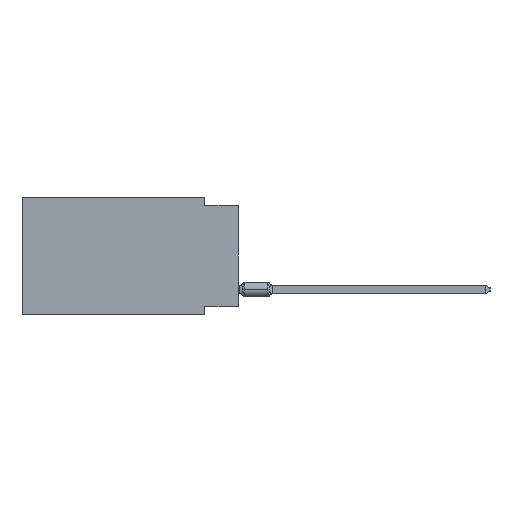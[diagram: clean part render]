
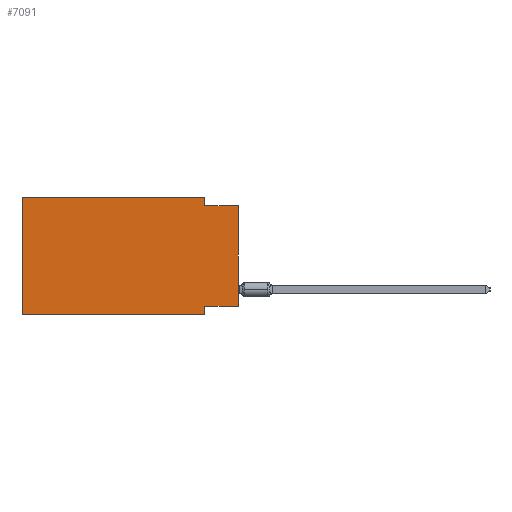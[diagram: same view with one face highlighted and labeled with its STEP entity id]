
A CAD part, left-side view. The second image highlights one B-rep face of the part: STEP entity #7091.
In plain terms, the highlighted planar face has unit normal (-1, 0, 0).
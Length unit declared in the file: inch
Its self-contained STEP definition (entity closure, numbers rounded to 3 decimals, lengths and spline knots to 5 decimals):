
#1363 = CARTESIAN_POINT ( 'NONE',  ( 0., 0., -0.325 ) ) ;
#2406 = DIRECTION ( 'NONE',  ( 0., 0., -1. ) ) ;
#4223 = EDGE_CURVE ( 'NONE', #99564, #10170, #31733, .T. ) ;
#4282 = LINE ( 'NONE', #84194, #91702 ) ;
#7091 = ADVANCED_FACE ( 'NONE', ( #85980 ), #93280, .F. ) ;
#7467 = CARTESIAN_POINT ( 'NONE',  ( 0., 0.645, 0. ) ) ;
#8281 = LINE ( 'NONE', #88220, #32033 ) ;
#8708 = EDGE_CURVE ( 'NONE', #79408, #15203, #8281, .T. ) ;
#10170 = VERTEX_POINT ( 'NONE', #73084 ) ;
#10191 = CARTESIAN_POINT ( 'NONE',  ( 0., 0.1, 0. ) ) ;
#11594 = CARTESIAN_POINT ( 'NONE',  ( 0., 0., 0. ) ) ;
#12178 = EDGE_CURVE ( 'NONE', #32904, #79408, #102466, .T. ) ;
#15203 = VERTEX_POINT ( 'NONE', #91053 ) ;
#17018 = VERTEX_POINT ( 'NONE', #29760 ) ;
#17642 = DIRECTION ( 'NONE',  ( 0., -1., 0. ) ) ;
#20343 = CARTESIAN_POINT ( 'NONE',  ( 0., 0.1, -0.025 ) ) ;
#28086 = VECTOR ( 'NONE', #47106, 39.37008 ) ;
#29302 = ORIENTED_EDGE ( 'NONE', *, *, #82862, .F. ) ;
#29760 = CARTESIAN_POINT ( 'NONE',  ( 0., 0.1, -0.325 ) ) ;
#31733 = LINE ( 'NONE', #101323, #88488 ) ;
#31818 = DIRECTION ( 'NONE',  ( 0., -1., 0. ) ) ;
#32033 = VECTOR ( 'NONE', #31818, 39.37008 ) ;
#32904 = VERTEX_POINT ( 'NONE', #97668 ) ;
#39822 = LINE ( 'NONE', #1363, #28086 ) ;
#40820 = ORIENTED_EDGE ( 'NONE', *, *, #8708, .F. ) ;
#44756 = DIRECTION ( 'NONE',  ( 0., 0., -1. ) ) ;
#45293 = ORIENTED_EDGE ( 'NONE', *, *, #4223, .F. ) ;
#47106 = DIRECTION ( 'NONE',  ( 0., 1., 0. ) ) ;
#51353 = EDGE_CURVE ( 'NONE', #32904, #85572, #88753, .T. ) ;
#53718 = EDGE_CURVE ( 'NONE', #17018, #85572, #4282, .T. ) ;
#54273 = ORIENTED_EDGE ( 'NONE', *, *, #85349, .T. ) ;
#63018 = DIRECTION ( 'NONE',  ( 0., 0., 1. ) ) ;
#63971 = ORIENTED_EDGE ( 'NONE', *, *, #53718, .F. ) ;
#66106 = DIRECTION ( 'NONE',  ( 0., 0., 1. ) ) ;
#66278 = LINE ( 'NONE', #10191, #70464 ) ;
#68367 = VECTOR ( 'NONE', #17642, 39.37008 ) ;
#68735 = CARTESIAN_POINT ( 'NONE',  ( 0., 0., -0.325 ) ) ;
#70464 = VECTOR ( 'NONE', #2406, 39.37008 ) ;
#70679 = DIRECTION ( 'NONE',  ( 0., -1., 0. ) ) ;
#70931 = CARTESIAN_POINT ( 'NONE',  ( 0., 0.645, 0. ) ) ;
#71447 = DIRECTION ( 'NONE',  ( 0., 0., -1. ) ) ;
#72074 = EDGE_CURVE ( 'NONE', #15203, #99564, #66278, .T. ) ;
#73084 = CARTESIAN_POINT ( 'NONE',  ( 0., 0., -0.025 ) ) ;
#78734 = ORIENTED_EDGE ( 'NONE', *, *, #51353, .T. ) ;
#79257 = ORIENTED_EDGE ( 'NONE', *, *, #72074, .F. ) ;
#79268 = VECTOR ( 'NONE', #63018, 39.37008 ) ;
#79408 = VERTEX_POINT ( 'NONE', #88078 ) ;
#81542 = AXIS2_PLACEMENT_3D ( 'NONE', #70931, #101584, #71447 ) ;
#82862 = EDGE_CURVE ( 'NONE', #100185, #17018, #39822, .T. ) ;
#84194 = CARTESIAN_POINT ( 'NONE',  ( 0., 0.1, -0.35 ) ) ;
#84884 = ORIENTED_EDGE ( 'NONE', *, *, #12178, .F. ) ;
#85349 = EDGE_CURVE ( 'NONE', #100185, #10170, #90498, .T. ) ;
#85572 = VERTEX_POINT ( 'NONE', #87794 ) ;
#85980 = FACE_OUTER_BOUND ( 'NONE', #99212, .T. ) ;
#87794 = CARTESIAN_POINT ( 'NONE',  ( 0., 0.1, -0.35 ) ) ;
#88078 = CARTESIAN_POINT ( 'NONE',  ( 0., 0.645, 0. ) ) ;
#88220 = CARTESIAN_POINT ( 'NONE',  ( 0., 0.645, 0. ) ) ;
#88488 = VECTOR ( 'NONE', #70679, 39.37008 ) ;
#88753 = LINE ( 'NONE', #94113, #68367 ) ;
#90498 = LINE ( 'NONE', #11594, #92894 ) ;
#91053 = CARTESIAN_POINT ( 'NONE',  ( 0., 0.1, 0. ) ) ;
#91702 = VECTOR ( 'NONE', #44756, 39.37008 ) ;
#92894 = VECTOR ( 'NONE', #66106, 39.37008 ) ;
#93280 = PLANE ( 'NONE',  #81542 ) ;
#94113 = CARTESIAN_POINT ( 'NONE',  ( 0., 0.645, -0.35 ) ) ;
#97668 = CARTESIAN_POINT ( 'NONE',  ( 0., 0.645, -0.35 ) ) ;
#99212 = EDGE_LOOP ( 'NONE', ( #54273, #45293, #79257, #40820, #84884, #78734, #63971, #29302 ) ) ;
#99564 = VERTEX_POINT ( 'NONE', #20343 ) ;
#100185 = VERTEX_POINT ( 'NONE', #68735 ) ;
#101323 = CARTESIAN_POINT ( 'NONE',  ( 0., 0., -0.025 ) ) ;
#101584 = DIRECTION ( 'NONE',  ( 1., 0., 0. ) ) ;
#102466 = LINE ( 'NONE', #7467, #79268 ) ;
